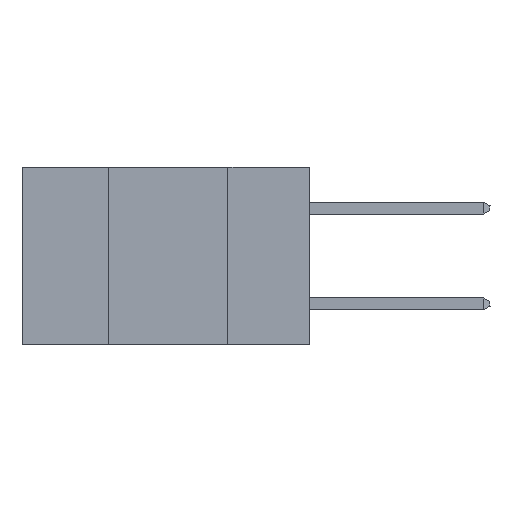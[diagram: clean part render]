
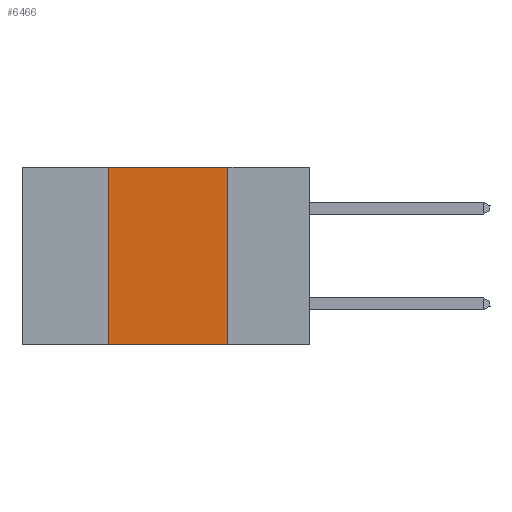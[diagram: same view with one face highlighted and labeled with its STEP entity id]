
A CAD part, left-side view. The second image highlights one B-rep face of the part: STEP entity #6466.
In plain terms, the highlighted planar face has unit normal (-1, 0, 0).
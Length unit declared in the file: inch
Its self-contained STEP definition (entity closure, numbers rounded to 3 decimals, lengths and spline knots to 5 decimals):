
#213 = EDGE_CURVE ( 'NONE', #14469, #8607, #13094, .T. ) ;
#496 = VECTOR ( 'NONE', #22061, 39.37008 ) ;
#608 = ORIENTED_EDGE ( 'NONE', *, *, #8600, .F. ) ;
#2525 = VECTOR ( 'NONE', #20848, 39.37008 ) ;
#2696 = LINE ( 'NONE', #6262, #11614 ) ;
#3084 = DIRECTION ( 'NONE',  ( 0., -1., 0. ) ) ;
#3680 = CARTESIAN_POINT ( 'NONE',  ( 0., 0.42, 0. ) ) ;
#4226 = LINE ( 'NONE', #15663, #2525 ) ;
#4544 = PLANE ( 'NONE',  #20574 ) ;
#5359 = LINE ( 'NONE', #13484, #496 ) ;
#5966 = CARTESIAN_POINT ( 'NONE',  ( 0., 0.6, -0.37 ) ) ;
#6262 = CARTESIAN_POINT ( 'NONE',  ( 0., 0.17, 0. ) ) ;
#6466 = ADVANCED_FACE ( 'NONE', ( #13595 ), #4544, .F. ) ;
#7298 = CARTESIAN_POINT ( 'NONE',  ( 0., 0.17, 0. ) ) ;
#7915 = CARTESIAN_POINT ( 'NONE',  ( 0., 0.42, -0.37 ) ) ;
#8600 = EDGE_CURVE ( 'NONE', #11080, #8607, #2696, .T. ) ;
#8607 = VERTEX_POINT ( 'NONE', #18340 ) ;
#10264 = VERTEX_POINT ( 'NONE', #3680 ) ;
#11080 = VERTEX_POINT ( 'NONE', #7298 ) ;
#11614 = VECTOR ( 'NONE', #13256, 39.37008 ) ;
#13094 = LINE ( 'NONE', #5966, #22154 ) ;
#13256 = DIRECTION ( 'NONE',  ( 0., 0., -1. ) ) ;
#13354 = ORIENTED_EDGE ( 'NONE', *, *, #17045, .F. ) ;
#13484 = CARTESIAN_POINT ( 'NONE',  ( 0., 0.42, 0. ) ) ;
#13513 = ORIENTED_EDGE ( 'NONE', *, *, #17190, .F. ) ;
#13595 = FACE_OUTER_BOUND ( 'NONE', #21554, .T. ) ;
#14469 = VERTEX_POINT ( 'NONE', #7915 ) ;
#15357 = CARTESIAN_POINT ( 'NONE',  ( 0., 0.6, 0. ) ) ;
#15663 = CARTESIAN_POINT ( 'NONE',  ( 0., 0.6, 0. ) ) ;
#17045 = EDGE_CURVE ( 'NONE', #14469, #10264, #5359, .T. ) ;
#17190 = EDGE_CURVE ( 'NONE', #10264, #11080, #4226, .T. ) ;
#18340 = CARTESIAN_POINT ( 'NONE',  ( 0., 0.17, -0.37 ) ) ;
#19614 = ORIENTED_EDGE ( 'NONE', *, *, #213, .T. ) ;
#20574 = AXIS2_PLACEMENT_3D ( 'NONE', #15357, #21588, #22311 ) ;
#20848 = DIRECTION ( 'NONE',  ( 0., -1., 0. ) ) ;
#21554 = EDGE_LOOP ( 'NONE', ( #608, #13513, #13354, #19614 ) ) ;
#21588 = DIRECTION ( 'NONE',  ( 1., 0., 0. ) ) ;
#22061 = DIRECTION ( 'NONE',  ( 0., 0., 1. ) ) ;
#22154 = VECTOR ( 'NONE', #3084, 39.37008 ) ;
#22311 = DIRECTION ( 'NONE',  ( 0., 0., -1. ) ) ;
